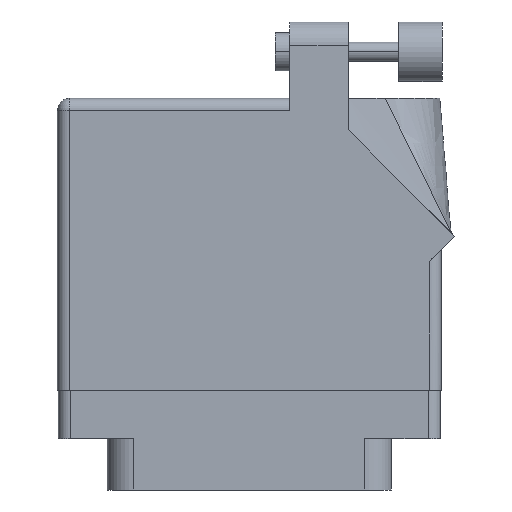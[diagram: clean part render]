
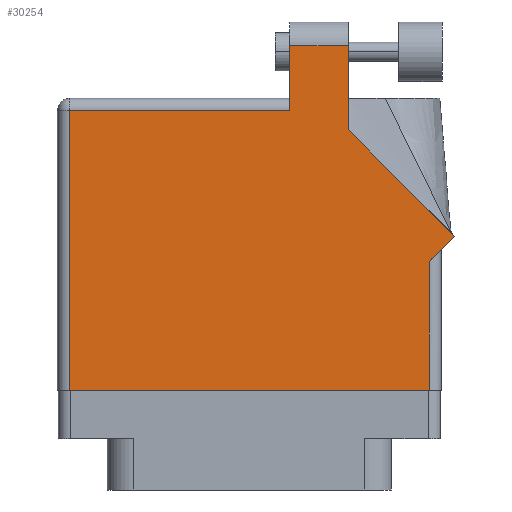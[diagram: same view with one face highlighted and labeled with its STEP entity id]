
A CAD part, front view. The second image highlights one B-rep face of the part: STEP entity #30254.
In plain terms, the highlighted face is planar.
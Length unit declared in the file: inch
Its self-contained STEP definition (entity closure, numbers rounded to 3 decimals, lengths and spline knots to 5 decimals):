
#513 = VERTEX_POINT ( 'NONE', #30731 ) ;
#671 = ORIENTED_EDGE ( 'NONE', *, *, #8275, .T. ) ;
#1051 = CARTESIAN_POINT ( 'NONE',  ( 0.212, 1.43, 0.455 ) ) ;
#1853 = CARTESIAN_POINT ( 'NONE',  ( 0.943, 0.575, 0.455 ) ) ;
#2049 = CARTESIAN_POINT ( 'NONE',  ( 0.212, 1.368, 0.455 ) ) ;
#2386 = CARTESIAN_POINT ( 'NONE',  ( 0.943, 0.637, 0.455 ) ) ;
#2390 = ORIENTED_EDGE ( 'NONE', *, *, #12453, .T. ) ;
#3079 = CARTESIAN_POINT ( 'NONE',  ( -1.005, 1.43, 0.455 ) ) ;
#3497 = FACE_OUTER_BOUND ( 'NONE', #19467, .T. ) ;
#4536 = EDGE_CURVE ( 'NONE', #30583, #37113, #8065, .T. ) ;
#4665 = DIRECTION ( 'NONE',  ( -1., 0., 0. ) ) ;
#5328 = ORIENTED_EDGE ( 'NONE', *, *, #4536, .T. ) ;
#5372 = LINE ( 'NONE', #30115, #30026 ) ;
#6389 = VECTOR ( 'NONE', #9881, 39.37008 ) ;
#7436 = CARTESIAN_POINT ( 'NONE',  ( 1.07571, 0.70771, 0.455 ) ) ;
#8065 = LINE ( 'NONE', #2386, #15340 ) ;
#8275 = EDGE_CURVE ( 'NONE', #12495, #17307, #32451, .T. ) ;
#8621 = DIRECTION ( 'NONE',  ( 0.707, 0.707, 0. ) ) ;
#9881 = DIRECTION ( 'NONE',  ( -0.707, 0.707, 0. ) ) ;
#10407 = EDGE_CURVE ( 'NONE', #17307, #24929, #17304, .T. ) ;
#10968 = VERTEX_POINT ( 'NONE', #27643 ) ;
#11627 = CARTESIAN_POINT ( 'NONE',  ( 0.212, 1.705, 0.455 ) ) ;
#12453 = EDGE_CURVE ( 'NONE', #513, #12495, #12808, .T. ) ;
#12495 = VERTEX_POINT ( 'NONE', #2049 ) ;
#12808 = LINE ( 'NONE', #1051, #34268 ) ;
#13218 = VECTOR ( 'NONE', #4665, 39.37008 ) ;
#13459 = EDGE_CURVE ( 'NONE', #10968, #28258, #34645, .T. ) ;
#13692 = LINE ( 'NONE', #7436, #6389 ) ;
#14467 = DIRECTION ( 'NONE',  ( 0., -1., 0. ) ) ;
#15340 = VECTOR ( 'NONE', #32614, 39.37008 ) ;
#15443 = DIRECTION ( 'NONE',  ( 0., 0., -1. ) ) ;
#15849 = PLANE ( 'NONE',  #39365 ) ;
#16395 = CARTESIAN_POINT ( 'NONE',  ( 1.07571, 0.70771, 0.455 ) ) ;
#16888 = DIRECTION ( 'NONE',  ( 1., 0., 0. ) ) ;
#16966 = ORIENTED_EDGE ( 'NONE', *, *, #26501, .T. ) ;
#17291 = CARTESIAN_POINT ( 'NONE',  ( -1.005, -0.1, 0.455 ) ) ;
#17304 = LINE ( 'NONE', #23632, #26361 ) ;
#17307 = VERTEX_POINT ( 'NONE', #26840 ) ;
#17336 = VECTOR ( 'NONE', #28559, 39.37008 ) ;
#17722 = DIRECTION ( 'NONE',  ( -1., 0., 0. ) ) ;
#17965 = ORIENTED_EDGE ( 'NONE', *, *, #24980, .T. ) ;
#19467 = EDGE_LOOP ( 'NONE', ( #38190, #17965, #2390, #671, #29959, #32213, #5328, #16966, #19760 ) ) ;
#19699 = DIRECTION ( 'NONE',  ( 0., -1., 0. ) ) ;
#19760 = ORIENTED_EDGE ( 'NONE', *, *, #32469, .T. ) ;
#22335 = EDGE_CURVE ( 'NONE', #24929, #30583, #38434, .T. ) ;
#22412 = VECTOR ( 'NONE', #16888, 39.37008 ) ;
#22454 = CARTESIAN_POINT ( 'NONE',  ( 0.519, 1.705, 0.455 ) ) ;
#23632 = CARTESIAN_POINT ( 'NONE',  ( -0.943, -0.1, 0.455 ) ) ;
#23829 = LINE ( 'NONE', #11627, #32539 ) ;
#24929 = VERTEX_POINT ( 'NONE', #39454 ) ;
#24980 = EDGE_CURVE ( 'NONE', #28258, #513, #23829, .T. ) ;
#25585 = CARTESIAN_POINT ( 'NONE',  ( -1.005, 1.368, 0.455 ) ) ;
#26361 = VECTOR ( 'NONE', #14467, 39.37008 ) ;
#26501 = EDGE_CURVE ( 'NONE', #37113, #31994, #5372, .T. ) ;
#26840 = CARTESIAN_POINT ( 'NONE',  ( -0.943, 1.368, 0.455 ) ) ;
#27643 = CARTESIAN_POINT ( 'NONE',  ( 0.519, 1.26442, 0.455 ) ) ;
#27841 = DIRECTION ( 'NONE',  ( -1., 0., 0. ) ) ;
#28200 = CARTESIAN_POINT ( 'NONE',  ( 0.943, -0.1, 0.455 ) ) ;
#28258 = VERTEX_POINT ( 'NONE', #22454 ) ;
#28365 = CARTESIAN_POINT ( 'NONE',  ( 0.519, 1.26442, 0.455 ) ) ;
#28559 = DIRECTION ( 'NONE',  ( 0., 1., 0. ) ) ;
#29959 = ORIENTED_EDGE ( 'NONE', *, *, #10407, .T. ) ;
#30026 = VECTOR ( 'NONE', #8621, 39.37008 ) ;
#30115 = CARTESIAN_POINT ( 'NONE',  ( 1.005, 0.637, 0.455 ) ) ;
#30254 = ADVANCED_FACE ( 'NONE', ( #3497 ), #15849, .F. ) ;
#30583 = VERTEX_POINT ( 'NONE', #28200 ) ;
#30731 = CARTESIAN_POINT ( 'NONE',  ( 0.212, 1.705, 0.455 ) ) ;
#31994 = VERTEX_POINT ( 'NONE', #16395 ) ;
#32213 = ORIENTED_EDGE ( 'NONE', *, *, #22335, .T. ) ;
#32451 = LINE ( 'NONE', #25585, #13218 ) ;
#32469 = EDGE_CURVE ( 'NONE', #31994, #10968, #13692, .T. ) ;
#32539 = VECTOR ( 'NONE', #17722, 39.37008 ) ;
#32614 = DIRECTION ( 'NONE',  ( 0., 1., 0. ) ) ;
#34268 = VECTOR ( 'NONE', #19699, 39.37008 ) ;
#34645 = LINE ( 'NONE', #28365, #17336 ) ;
#37113 = VERTEX_POINT ( 'NONE', #1853 ) ;
#38190 = ORIENTED_EDGE ( 'NONE', *, *, #13459, .T. ) ;
#38434 = LINE ( 'NONE', #17291, #22412 ) ;
#39365 = AXIS2_PLACEMENT_3D ( 'NONE', #3079, #15443, #27841 ) ;
#39454 = CARTESIAN_POINT ( 'NONE',  ( -0.943, -0.1, 0.455 ) ) ;
